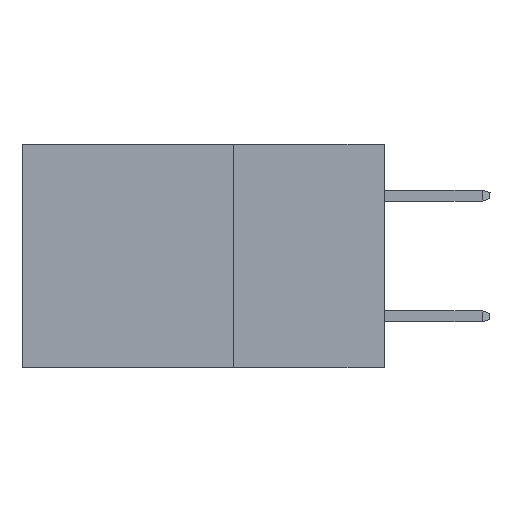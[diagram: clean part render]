
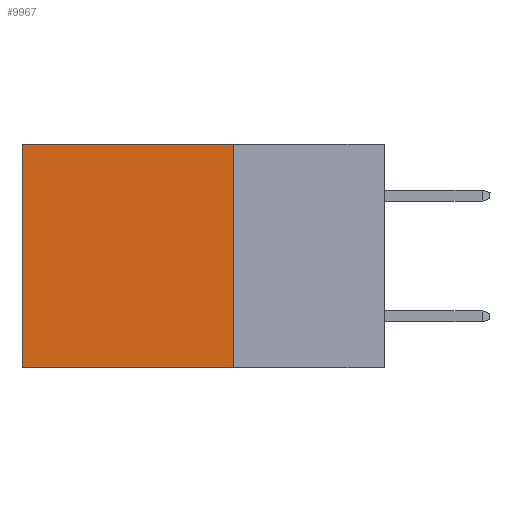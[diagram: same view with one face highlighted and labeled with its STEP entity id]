
A CAD part, left-side view. The second image highlights one B-rep face of the part: STEP entity #9967.
In plain terms, the highlighted planar face has unit normal (-1, 0, 0).
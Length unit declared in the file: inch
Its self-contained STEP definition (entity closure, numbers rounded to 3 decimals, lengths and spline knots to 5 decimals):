
#15 = CARTESIAN_POINT ( 'NONE',  ( 0.298, 0.6, 0. ) ) ;
#1397 = ORIENTED_EDGE ( 'NONE', *, *, #22311, .T. ) ;
#1519 = EDGE_CURVE ( 'NONE', #23626, #3024, #4407, .T. ) ;
#2277 = DIRECTION ( 'NONE',  ( 0., 0., -1. ) ) ;
#2551 = VECTOR ( 'NONE', #7333, 39.37008 ) ;
#3024 = VERTEX_POINT ( 'NONE', #27278 ) ;
#3601 = VERTEX_POINT ( 'NONE', #24641 ) ;
#3767 = EDGE_CURVE ( 'NONE', #3601, #18844, #6139, .T. ) ;
#4407 = LINE ( 'NONE', #15, #17342 ) ;
#5854 = ORIENTED_EDGE ( 'NONE', *, *, #1519, .T. ) ;
#6139 = LINE ( 'NONE', #22755, #19373 ) ;
#6546 = ORIENTED_EDGE ( 'NONE', *, *, #26808, .F. ) ;
#6622 = VECTOR ( 'NONE', #17281, 39.37008 ) ;
#7333 = DIRECTION ( 'NONE',  ( 0., 1., 0. ) ) ;
#7473 = DIRECTION ( 'NONE',  ( 0., 0., -1. ) ) ;
#8766 = ORIENTED_EDGE ( 'NONE', *, *, #3767, .F. ) ;
#9845 = EDGE_LOOP ( 'NONE', ( #5854, #6546, #8766, #1397 ) ) ;
#9858 = DIRECTION ( 'NONE',  ( 1., 0., 0. ) ) ;
#9967 = ADVANCED_FACE ( 'NONE', ( #12472 ), #15860, .F. ) ;
#10928 = CARTESIAN_POINT ( 'NONE',  ( 0.298, 0.25, -0.37 ) ) ;
#11568 = CARTESIAN_POINT ( 'NONE',  ( 0.298, 0.25, 0. ) ) ;
#12472 = FACE_OUTER_BOUND ( 'NONE', #9845, .T. ) ;
#13789 = LINE ( 'NONE', #17565, #6622 ) ;
#14860 = AXIS2_PLACEMENT_3D ( 'NONE', #11568, #9858, #22223 ) ;
#15860 = PLANE ( 'NONE',  #14860 ) ;
#17281 = DIRECTION ( 'NONE',  ( 0., 1., 0. ) ) ;
#17342 = VECTOR ( 'NONE', #2277, 39.37008 ) ;
#17565 = CARTESIAN_POINT ( 'NONE',  ( 0.298, 0.25, -0.37 ) ) ;
#18474 = CARTESIAN_POINT ( 'NONE',  ( 0.298, 0.25, 0. ) ) ;
#18844 = VERTEX_POINT ( 'NONE', #10928 ) ;
#19373 = VECTOR ( 'NONE', #7473, 39.37008 ) ;
#21471 = CARTESIAN_POINT ( 'NONE',  ( 0.298, 0.6, 0. ) ) ;
#22223 = DIRECTION ( 'NONE',  ( 0., 0., -1. ) ) ;
#22311 = EDGE_CURVE ( 'NONE', #3601, #23626, #26617, .T. ) ;
#22755 = CARTESIAN_POINT ( 'NONE',  ( 0.298, 0.25, 0. ) ) ;
#23626 = VERTEX_POINT ( 'NONE', #21471 ) ;
#24641 = CARTESIAN_POINT ( 'NONE',  ( 0.298, 0.25, 0. ) ) ;
#26617 = LINE ( 'NONE', #18474, #2551 ) ;
#26808 = EDGE_CURVE ( 'NONE', #18844, #3024, #13789, .T. ) ;
#27278 = CARTESIAN_POINT ( 'NONE',  ( 0.298, 0.6, -0.37 ) ) ;
